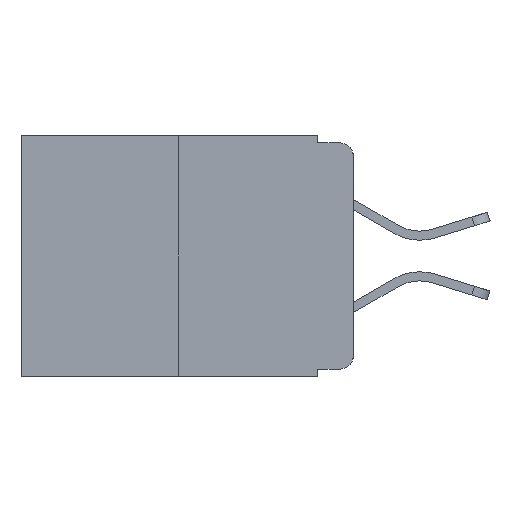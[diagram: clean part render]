
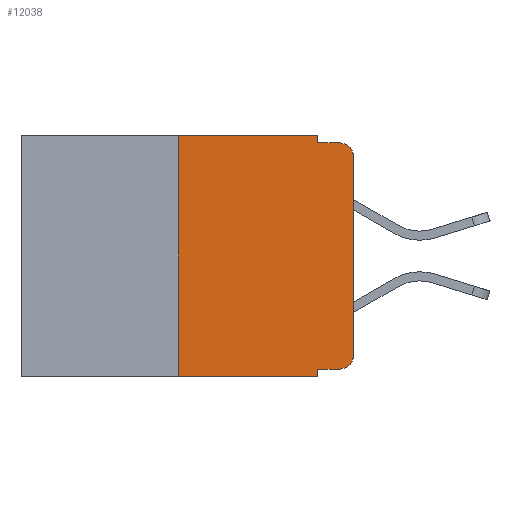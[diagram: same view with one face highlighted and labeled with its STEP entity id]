
A CAD part, left-side view. The second image highlights one B-rep face of the part: STEP entity #12038.
In plain terms, the highlighted planar face has unit normal (-1, 0, 0).
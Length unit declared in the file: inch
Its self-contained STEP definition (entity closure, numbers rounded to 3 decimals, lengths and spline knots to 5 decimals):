
#293 = CIRCLE ( 'NONE', #12383, 0.02 ) ;
#406 = CARTESIAN_POINT ( 'NONE',  ( 0., 0., 0. ) ) ;
#571 = DIRECTION ( 'NONE',  ( 0., -1., 0. ) ) ;
#690 = CARTESIAN_POINT ( 'NONE',  ( 0., 0.02, -0.03 ) ) ;
#748 = LINE ( 'NONE', #6248, #10760 ) ;
#876 = EDGE_CURVE ( 'NONE', #5214, #4061, #12280, .T. ) ;
#2083 = DIRECTION ( 'NONE',  ( 0., 0., -1. ) ) ;
#2453 = LINE ( 'NONE', #4392, #11143 ) ;
#2536 = AXIS2_PLACEMENT_3D ( 'NONE', #3546, #15125, #7462 ) ;
#2737 = LINE ( 'NONE', #11428, #8796 ) ;
#2867 = ORIENTED_EDGE ( 'NONE', *, *, #16427, .F. ) ;
#2977 = VERTEX_POINT ( 'NONE', #13901 ) ;
#3136 = CARTESIAN_POINT ( 'NONE',  ( 0., 0.473, 0. ) ) ;
#3290 = ORIENTED_EDGE ( 'NONE', *, *, #10744, .T. ) ;
#3400 = CARTESIAN_POINT ( 'NONE',  ( 0., 0.051, -0.333 ) ) ;
#3546 = CARTESIAN_POINT ( 'NONE',  ( 0., 0.473, 0. ) ) ;
#3654 = EDGE_LOOP ( 'NONE', ( #14820, #4244, #2867, #7867, #12750, #5896, #3290, #16276, #15899, #9935 ) ) ;
#3681 = DIRECTION ( 'NONE',  ( 0., 0., -1. ) ) ;
#3834 = AXIS2_PLACEMENT_3D ( 'NONE', #5371, #14360, #6665 ) ;
#3971 = EDGE_CURVE ( 'NONE', #2977, #12426, #12367, .T. ) ;
#4061 = VERTEX_POINT ( 'NONE', #9731 ) ;
#4092 = EDGE_CURVE ( 'NONE', #15507, #6483, #293, .T. ) ;
#4244 = ORIENTED_EDGE ( 'NONE', *, *, #4092, .T. ) ;
#4375 = LINE ( 'NONE', #5188, #13839 ) ;
#4392 = CARTESIAN_POINT ( 'NONE',  ( 0., 0.051, -0.01 ) ) ;
#5188 = CARTESIAN_POINT ( 'NONE',  ( 0., 0.25, 0. ) ) ;
#5214 = VERTEX_POINT ( 'NONE', #13986 ) ;
#5371 = CARTESIAN_POINT ( 'NONE',  ( 0., 0.02, -0.313 ) ) ;
#5425 = VECTOR ( 'NONE', #7401, 39.37008 ) ;
#5896 = ORIENTED_EDGE ( 'NONE', *, *, #12202, .F. ) ;
#5901 = VECTOR ( 'NONE', #12147, 39.37008 ) ;
#6134 = PLANE ( 'NONE',  #2536 ) ;
#6149 = EDGE_CURVE ( 'NONE', #5214, #13182, #2737, .T. ) ;
#6248 = CARTESIAN_POINT ( 'NONE',  ( 0., 0.051, 0. ) ) ;
#6331 = LINE ( 'NONE', #406, #16524 ) ;
#6409 = FACE_OUTER_BOUND ( 'NONE', #3654, .T. ) ;
#6483 = VERTEX_POINT ( 'NONE', #6943 ) ;
#6653 = CARTESIAN_POINT ( 'NONE',  ( 0., 0., -0.313 ) ) ;
#6665 = DIRECTION ( 'NONE',  ( 0., 0., -1. ) ) ;
#6943 = CARTESIAN_POINT ( 'NONE',  ( 0., 0.02, -0.01 ) ) ;
#6981 = VERTEX_POINT ( 'NONE', #13004 ) ;
#7352 = CARTESIAN_POINT ( 'NONE',  ( 0., 0., -0.03 ) ) ;
#7401 = DIRECTION ( 'NONE',  ( 0., -1., 0. ) ) ;
#7462 = DIRECTION ( 'NONE',  ( 0., 0., -1. ) ) ;
#7596 = EDGE_CURVE ( 'NONE', #8191, #15507, #6331, .T. ) ;
#7867 = ORIENTED_EDGE ( 'NONE', *, *, #15603, .F. ) ;
#8191 = VERTEX_POINT ( 'NONE', #6653 ) ;
#8471 = LINE ( 'NONE', #16068, #14857 ) ;
#8796 = VECTOR ( 'NONE', #3681, 39.37008 ) ;
#9050 = CIRCLE ( 'NONE', #3834, 0.02 ) ;
#9731 = CARTESIAN_POINT ( 'NONE',  ( 0., 0.02, -0.333 ) ) ;
#9840 = DIRECTION ( 'NONE',  ( -1., 0., 0. ) ) ;
#9935 = ORIENTED_EDGE ( 'NONE', *, *, #13375, .T. ) ;
#10380 = DIRECTION ( 'NONE',  ( 0., 0., 1. ) ) ;
#10744 = EDGE_CURVE ( 'NONE', #14959, #13182, #8471, .T. ) ;
#10760 = VECTOR ( 'NONE', #13950, 39.37008 ) ;
#11143 = VECTOR ( 'NONE', #13408, 39.37008 ) ;
#11428 = CARTESIAN_POINT ( 'NONE',  ( 0., 0.051, 0. ) ) ;
#12038 = ADVANCED_FACE ( 'NONE', ( #6409 ), #6134, .F. ) ;
#12147 = DIRECTION ( 'NONE',  ( 0., -1., 0. ) ) ;
#12202 = EDGE_CURVE ( 'NONE', #14959, #2977, #4375, .T. ) ;
#12280 = LINE ( 'NONE', #3400, #5425 ) ;
#12367 = LINE ( 'NONE', #3136, #5901 ) ;
#12383 = AXIS2_PLACEMENT_3D ( 'NONE', #690, #9840, #2083 ) ;
#12415 = CARTESIAN_POINT ( 'NONE',  ( 0., 0.25, -0.343 ) ) ;
#12426 = VERTEX_POINT ( 'NONE', #13384 ) ;
#12709 = CARTESIAN_POINT ( 'NONE',  ( 0., 0.051, -0.343 ) ) ;
#12750 = ORIENTED_EDGE ( 'NONE', *, *, #3971, .F. ) ;
#13004 = CARTESIAN_POINT ( 'NONE',  ( 0., 0.051, -0.01 ) ) ;
#13030 = DIRECTION ( 'NONE',  ( 0., 0., 1. ) ) ;
#13182 = VERTEX_POINT ( 'NONE', #12709 ) ;
#13375 = EDGE_CURVE ( 'NONE', #4061, #8191, #9050, .T. ) ;
#13384 = CARTESIAN_POINT ( 'NONE',  ( 0., 0.051, 0. ) ) ;
#13408 = DIRECTION ( 'NONE',  ( 0., -1., 0. ) ) ;
#13839 = VECTOR ( 'NONE', #10380, 39.37008 ) ;
#13901 = CARTESIAN_POINT ( 'NONE',  ( 0., 0.25, 0. ) ) ;
#13950 = DIRECTION ( 'NONE',  ( 0., 0., -1. ) ) ;
#13986 = CARTESIAN_POINT ( 'NONE',  ( 0., 0.051, -0.333 ) ) ;
#14360 = DIRECTION ( 'NONE',  ( -1., 0., 0. ) ) ;
#14820 = ORIENTED_EDGE ( 'NONE', *, *, #7596, .T. ) ;
#14857 = VECTOR ( 'NONE', #571, 39.37008 ) ;
#14959 = VERTEX_POINT ( 'NONE', #12415 ) ;
#15125 = DIRECTION ( 'NONE',  ( 1., 0., 0. ) ) ;
#15507 = VERTEX_POINT ( 'NONE', #7352 ) ;
#15603 = EDGE_CURVE ( 'NONE', #12426, #6981, #748, .T. ) ;
#15899 = ORIENTED_EDGE ( 'NONE', *, *, #876, .T. ) ;
#16068 = CARTESIAN_POINT ( 'NONE',  ( 0., 0.473, -0.343 ) ) ;
#16276 = ORIENTED_EDGE ( 'NONE', *, *, #6149, .F. ) ;
#16427 = EDGE_CURVE ( 'NONE', #6981, #6483, #2453, .T. ) ;
#16524 = VECTOR ( 'NONE', #13030, 39.37008 ) ;
